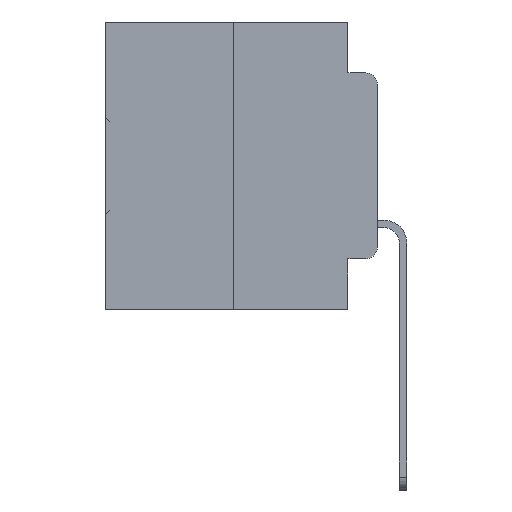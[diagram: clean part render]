
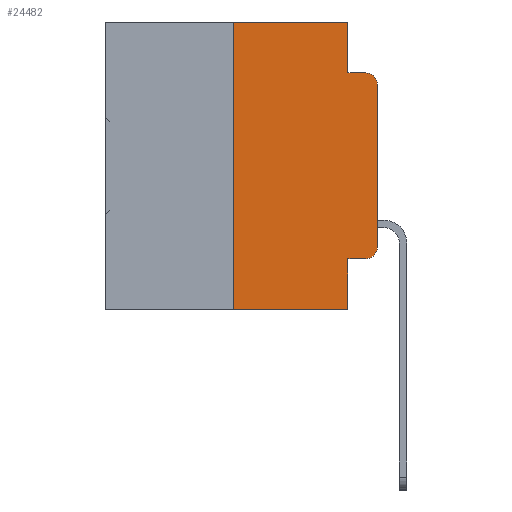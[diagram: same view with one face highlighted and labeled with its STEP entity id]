
A CAD part, left-side view. The second image highlights one B-rep face of the part: STEP entity #24482.
In plain terms, the highlighted planar face has unit normal (-1, 0, 0).
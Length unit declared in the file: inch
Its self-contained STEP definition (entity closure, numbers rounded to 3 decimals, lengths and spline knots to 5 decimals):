
#1528 = EDGE_CURVE ( 'NONE', #6294, #2712, #22273, .T. ) ;
#1926 = ORIENTED_EDGE ( 'NONE', *, *, #35772, .F. ) ;
#2400 = CARTESIAN_POINT ( 'NONE',  ( 0., 0.051, -0.0885 ) ) ;
#2712 = VERTEX_POINT ( 'NONE', #36366 ) ;
#2917 = EDGE_LOOP ( 'NONE', ( #5111, #20764, #1926, #9104, #10907, #34186, #31163, #19857, #24205, #25949 ) ) ;
#3498 = VERTEX_POINT ( 'NONE', #22003 ) ;
#3674 = CARTESIAN_POINT ( 'NONE',  ( 0., 0., -0.3915 ) ) ;
#3789 = VERTEX_POINT ( 'NONE', #31568 ) ;
#3826 = VERTEX_POINT ( 'NONE', #34466 ) ;
#3871 = VECTOR ( 'NONE', #23637, 39.37008 ) ;
#4427 = VERTEX_POINT ( 'NONE', #20359 ) ;
#4441 = VECTOR ( 'NONE', #33424, 39.37008 ) ;
#4728 = LINE ( 'NONE', #12733, #12293 ) ;
#4899 = EDGE_CURVE ( 'NONE', #24308, #3498, #35076, .T. ) ;
#4925 = LINE ( 'NONE', #20398, #26622 ) ;
#5111 = ORIENTED_EDGE ( 'NONE', *, *, #6798, .T. ) ;
#6294 = VERTEX_POINT ( 'NONE', #34825 ) ;
#6428 = AXIS2_PLACEMENT_3D ( 'NONE', #14502, #34107, #17411 ) ;
#6798 = EDGE_CURVE ( 'NONE', #20543, #24308, #25230, .T. ) ;
#8569 = VECTOR ( 'NONE', #30710, 39.37008 ) ;
#9104 = ORIENTED_EDGE ( 'NONE', *, *, #33925, .F. ) ;
#9485 = LINE ( 'NONE', #2400, #8569 ) ;
#9679 = VERTEX_POINT ( 'NONE', #14886 ) ;
#10056 = VECTOR ( 'NONE', #32119, 39.37008 ) ;
#10218 = VECTOR ( 'NONE', #25912, 39.37008 ) ;
#10364 = CARTESIAN_POINT ( 'NONE',  ( 0., 0.02, -0.4115 ) ) ;
#10907 = ORIENTED_EDGE ( 'NONE', *, *, #22806, .F. ) ;
#11060 = CARTESIAN_POINT ( 'NONE',  ( 0., 0.051, -0.4115 ) ) ;
#11084 = DIRECTION ( 'NONE',  ( -1., 0., 0. ) ) ;
#12293 = VECTOR ( 'NONE', #32415, 39.37008 ) ;
#12733 = CARTESIAN_POINT ( 'NONE',  ( 0., 0.051, 0. ) ) ;
#13289 = DIRECTION ( 'NONE',  ( 1., 0., 0. ) ) ;
#14136 = LINE ( 'NONE', #11060, #28251 ) ;
#14502 = CARTESIAN_POINT ( 'NONE',  ( 0., 0.02, -0.3915 ) ) ;
#14886 = CARTESIAN_POINT ( 'NONE',  ( 0., 0.25, 0. ) ) ;
#16685 = CARTESIAN_POINT ( 'NONE',  ( 0., 0.473, -0.5 ) ) ;
#17411 = DIRECTION ( 'NONE',  ( 0., 0., -1. ) ) ;
#17763 = FACE_OUTER_BOUND ( 'NONE', #2917, .T. ) ;
#18112 = VERTEX_POINT ( 'NONE', #10364 ) ;
#19857 = ORIENTED_EDGE ( 'NONE', *, *, #26471, .F. ) ;
#20359 = CARTESIAN_POINT ( 'NONE',  ( 0., 0.051, -0.0885 ) ) ;
#20398 = CARTESIAN_POINT ( 'NONE',  ( 0., 0.473, 0. ) ) ;
#20543 = VERTEX_POINT ( 'NONE', #3674 ) ;
#20764 = ORIENTED_EDGE ( 'NONE', *, *, #4899, .T. ) ;
#21307 = AXIS2_PLACEMENT_3D ( 'NONE', #30148, #13289, #32938 ) ;
#22003 = CARTESIAN_POINT ( 'NONE',  ( 0., 0.02, -0.0885 ) ) ;
#22273 = LINE ( 'NONE', #16685, #4441 ) ;
#22754 = EDGE_CURVE ( 'NONE', #18112, #20543, #30979, .T. ) ;
#22806 = EDGE_CURVE ( 'NONE', #9679, #3789, #4925, .T. ) ;
#23144 = CARTESIAN_POINT ( 'NONE',  ( 0., 0., 0. ) ) ;
#23178 = DIRECTION ( 'NONE',  ( 0., -1., 0. ) ) ;
#23637 = DIRECTION ( 'NONE',  ( 0., 0., 1. ) ) ;
#24205 = ORIENTED_EDGE ( 'NONE', *, *, #24582, .T. ) ;
#24308 = VERTEX_POINT ( 'NONE', #29440 ) ;
#24482 = ADVANCED_FACE ( 'NONE', ( #17763 ), #24527, .F. ) ;
#24527 = PLANE ( 'NONE',  #21307 ) ;
#24582 = EDGE_CURVE ( 'NONE', #3826, #18112, #14136, .T. ) ;
#25079 = LINE ( 'NONE', #29332, #10056 ) ;
#25230 = LINE ( 'NONE', #23144, #10218 ) ;
#25912 = DIRECTION ( 'NONE',  ( 0., 0., 1. ) ) ;
#25949 = ORIENTED_EDGE ( 'NONE', *, *, #22754, .T. ) ;
#26471 = EDGE_CURVE ( 'NONE', #3826, #2712, #25079, .T. ) ;
#26498 = LINE ( 'NONE', #34692, #3871 ) ;
#26622 = VECTOR ( 'NONE', #23178, 39.37008 ) ;
#27979 = CARTESIAN_POINT ( 'NONE',  ( 0., 0.02, -0.1085 ) ) ;
#28251 = VECTOR ( 'NONE', #33539, 39.37008 ) ;
#29231 = AXIS2_PLACEMENT_3D ( 'NONE', #27979, #11084, #30768 ) ;
#29332 = CARTESIAN_POINT ( 'NONE',  ( 0., 0.051, 0. ) ) ;
#29440 = CARTESIAN_POINT ( 'NONE',  ( 0., 0., -0.1085 ) ) ;
#30148 = CARTESIAN_POINT ( 'NONE',  ( 0., 0.473, 0. ) ) ;
#30710 = DIRECTION ( 'NONE',  ( 0., -1., 0. ) ) ;
#30768 = DIRECTION ( 'NONE',  ( 0., 0., -1. ) ) ;
#30979 = CIRCLE ( 'NONE', #6428, 0.02 ) ;
#31163 = ORIENTED_EDGE ( 'NONE', *, *, #1528, .T. ) ;
#31568 = CARTESIAN_POINT ( 'NONE',  ( 0., 0.051, 0. ) ) ;
#32070 = EDGE_CURVE ( 'NONE', #6294, #9679, #26498, .T. ) ;
#32119 = DIRECTION ( 'NONE',  ( 0., 0., -1. ) ) ;
#32415 = DIRECTION ( 'NONE',  ( 0., 0., -1. ) ) ;
#32938 = DIRECTION ( 'NONE',  ( 0., 0., -1. ) ) ;
#33424 = DIRECTION ( 'NONE',  ( 0., -1., 0. ) ) ;
#33539 = DIRECTION ( 'NONE',  ( 0., -1., 0. ) ) ;
#33925 = EDGE_CURVE ( 'NONE', #3789, #4427, #4728, .T. ) ;
#34107 = DIRECTION ( 'NONE',  ( -1., 0., 0. ) ) ;
#34186 = ORIENTED_EDGE ( 'NONE', *, *, #32070, .F. ) ;
#34466 = CARTESIAN_POINT ( 'NONE',  ( 0., 0.051, -0.4115 ) ) ;
#34692 = CARTESIAN_POINT ( 'NONE',  ( 0., 0.25, 0. ) ) ;
#34825 = CARTESIAN_POINT ( 'NONE',  ( 0., 0.25, -0.5 ) ) ;
#35076 = CIRCLE ( 'NONE', #29231, 0.02 ) ;
#35772 = EDGE_CURVE ( 'NONE', #4427, #3498, #9485, .T. ) ;
#36366 = CARTESIAN_POINT ( 'NONE',  ( 0., 0.051, -0.5 ) ) ;
